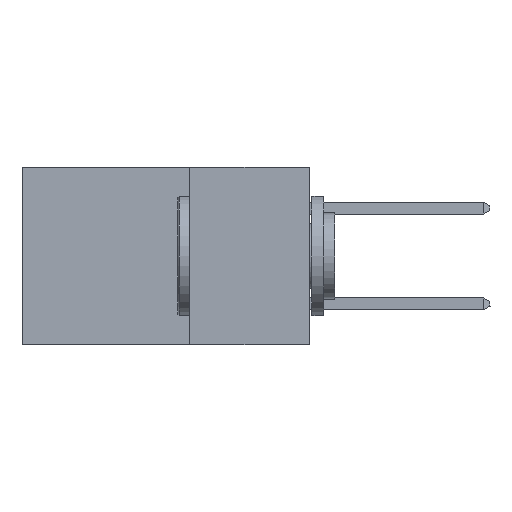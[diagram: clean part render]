
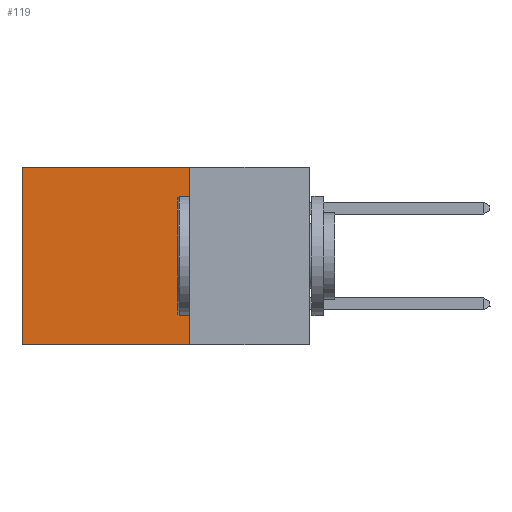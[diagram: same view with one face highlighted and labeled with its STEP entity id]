
A CAD part, left-side view. The second image highlights one B-rep face of the part: STEP entity #119.
In plain terms, the highlighted planar face has unit normal (-1, 0, 0).
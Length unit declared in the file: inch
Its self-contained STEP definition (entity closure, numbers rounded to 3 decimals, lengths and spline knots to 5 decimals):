
#119 = ADVANCED_FACE ( 'NONE', ( #18625 ), #8488, .F. ) ;
#2096 = DIRECTION ( 'NONE',  ( 0., 1., 0. ) ) ;
#3604 = EDGE_LOOP ( 'NONE', ( #32818, #21208, #25456, #25927 ) ) ;
#3654 = VERTEX_POINT ( 'NONE', #10963 ) ;
#4889 = VERTEX_POINT ( 'NONE', #12794 ) ;
#5588 = LINE ( 'NONE', #6343, #7582 ) ;
#6343 = CARTESIAN_POINT ( 'NONE',  ( 0.2875, 0.25, 0. ) ) ;
#7226 = VECTOR ( 'NONE', #20958, 39.37008 ) ;
#7457 = VECTOR ( 'NONE', #2096, 39.37008 ) ;
#7582 = VECTOR ( 'NONE', #19251, 39.37008 ) ;
#8487 = EDGE_CURVE ( 'NONE', #31371, #4889, #25855, .T. ) ;
#8488 = PLANE ( 'NONE',  #22349 ) ;
#10963 = CARTESIAN_POINT ( 'NONE',  ( 0.2875, 0.25, -0.37 ) ) ;
#11883 = CARTESIAN_POINT ( 'NONE',  ( 0.2875, 0.25, 0. ) ) ;
#12794 = CARTESIAN_POINT ( 'NONE',  ( 0.2875, 0.6, -0.37 ) ) ;
#13530 = EDGE_CURVE ( 'NONE', #3654, #4889, #21500, .T. ) ;
#14805 = DIRECTION ( 'NONE',  ( 0., 1., 0. ) ) ;
#18625 = FACE_OUTER_BOUND ( 'NONE', #3604, .T. ) ;
#19251 = DIRECTION ( 'NONE',  ( 0., 0., -1. ) ) ;
#20958 = DIRECTION ( 'NONE',  ( 0., 0., -1. ) ) ;
#21134 = DIRECTION ( 'NONE',  ( 1., 0., 0. ) ) ;
#21208 = ORIENTED_EDGE ( 'NONE', *, *, #13530, .F. ) ;
#21500 = LINE ( 'NONE', #27600, #7457 ) ;
#22349 = AXIS2_PLACEMENT_3D ( 'NONE', #27855, #21134, #27576 ) ;
#22741 = CARTESIAN_POINT ( 'NONE',  ( 0.2875, 0.25, 0. ) ) ;
#25456 = ORIENTED_EDGE ( 'NONE', *, *, #38380, .F. ) ;
#25855 = LINE ( 'NONE', #33852, #7226 ) ;
#25927 = ORIENTED_EDGE ( 'NONE', *, *, #33470, .T. ) ;
#27576 = DIRECTION ( 'NONE',  ( 0., 0., -1. ) ) ;
#27600 = CARTESIAN_POINT ( 'NONE',  ( 0.2875, 0.25, -0.37 ) ) ;
#27855 = CARTESIAN_POINT ( 'NONE',  ( 0.2875, 0.25, 0. ) ) ;
#31371 = VERTEX_POINT ( 'NONE', #37339 ) ;
#32112 = LINE ( 'NONE', #11883, #34609 ) ;
#32818 = ORIENTED_EDGE ( 'NONE', *, *, #8487, .T. ) ;
#33470 = EDGE_CURVE ( 'NONE', #35043, #31371, #32112, .T. ) ;
#33852 = CARTESIAN_POINT ( 'NONE',  ( 0.2875, 0.6, 0. ) ) ;
#34609 = VECTOR ( 'NONE', #14805, 39.37008 ) ;
#35043 = VERTEX_POINT ( 'NONE', #22741 ) ;
#37339 = CARTESIAN_POINT ( 'NONE',  ( 0.2875, 0.6, 0. ) ) ;
#38380 = EDGE_CURVE ( 'NONE', #35043, #3654, #5588, .T. ) ;
